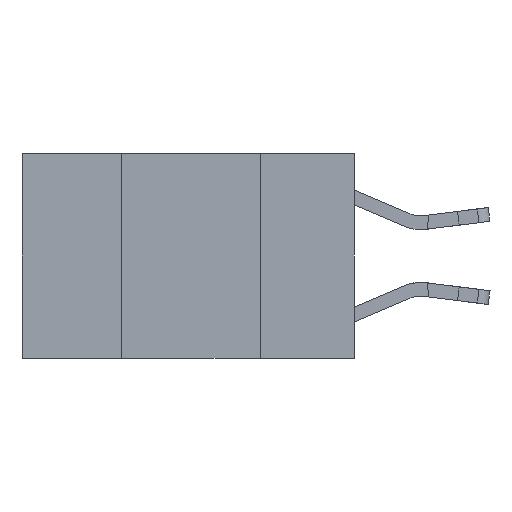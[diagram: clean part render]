
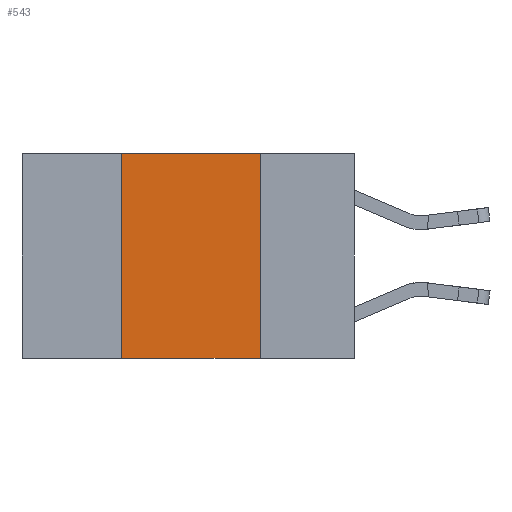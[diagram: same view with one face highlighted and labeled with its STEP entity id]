
A CAD part, left-side view. The second image highlights one B-rep face of the part: STEP entity #543.
In plain terms, the highlighted planar face has unit normal (-1, 0, 0).
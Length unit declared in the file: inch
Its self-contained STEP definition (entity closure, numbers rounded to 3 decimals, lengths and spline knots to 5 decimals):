
#543 = ADVANCED_FACE ( 'NONE', ( #21779 ), #15109, .F. ) ;
#1077 = CARTESIAN_POINT ( 'NONE',  ( 0., 0.42, -0.37 ) ) ;
#1255 = CARTESIAN_POINT ( 'NONE',  ( 0., 0.42, 0. ) ) ;
#1808 = LINE ( 'NONE', #9830, #12783 ) ;
#3515 = DIRECTION ( 'NONE',  ( 0., 0., -1. ) ) ;
#4391 = VECTOR ( 'NONE', #8949, 39.37008 ) ;
#5004 = VERTEX_POINT ( 'NONE', #21701 ) ;
#8763 = DIRECTION ( 'NONE',  ( 0., -1., 0. ) ) ;
#8823 = VERTEX_POINT ( 'NONE', #22672 ) ;
#8858 = CARTESIAN_POINT ( 'NONE',  ( 0., 0.42, 0. ) ) ;
#8949 = DIRECTION ( 'NONE',  ( 0., 0., 1. ) ) ;
#9587 = EDGE_CURVE ( 'NONE', #20659, #5004, #15775, .T. ) ;
#9830 = CARTESIAN_POINT ( 'NONE',  ( 0., 0.17, 0. ) ) ;
#10849 = CARTESIAN_POINT ( 'NONE',  ( 0., 0.6, -0.37 ) ) ;
#11234 = EDGE_LOOP ( 'NONE', ( #11750, #12379, #17799, #13031 ) ) ;
#11750 = ORIENTED_EDGE ( 'NONE', *, *, #12477, .F. ) ;
#12379 = ORIENTED_EDGE ( 'NONE', *, *, #22537, .F. ) ;
#12477 = EDGE_CURVE ( 'NONE', #8823, #5004, #1808, .T. ) ;
#12783 = VECTOR ( 'NONE', #3515, 39.37008 ) ;
#13031 = ORIENTED_EDGE ( 'NONE', *, *, #9587, .T. ) ;
#15109 = PLANE ( 'NONE',  #18834 ) ;
#15480 = CARTESIAN_POINT ( 'NONE',  ( 0., 0.6, 0. ) ) ;
#15775 = LINE ( 'NONE', #10849, #24631 ) ;
#15976 = LINE ( 'NONE', #8858, #4391 ) ;
#16313 = DIRECTION ( 'NONE',  ( 1., 0., 0. ) ) ;
#16536 = DIRECTION ( 'NONE',  ( 0., 0., -1. ) ) ;
#17236 = EDGE_CURVE ( 'NONE', #20659, #22680, #15976, .T. ) ;
#17799 = ORIENTED_EDGE ( 'NONE', *, *, #17236, .F. ) ;
#18834 = AXIS2_PLACEMENT_3D ( 'NONE', #15480, #16313, #16536 ) ;
#20659 = VERTEX_POINT ( 'NONE', #1077 ) ;
#21701 = CARTESIAN_POINT ( 'NONE',  ( 0., 0.17, -0.37 ) ) ;
#21779 = FACE_OUTER_BOUND ( 'NONE', #11234, .T. ) ;
#22537 = EDGE_CURVE ( 'NONE', #22680, #8823, #24919, .T. ) ;
#22672 = CARTESIAN_POINT ( 'NONE',  ( 0., 0.17, 0. ) ) ;
#22680 = VERTEX_POINT ( 'NONE', #1255 ) ;
#23354 = CARTESIAN_POINT ( 'NONE',  ( 0., 0.6, 0. ) ) ;
#24295 = VECTOR ( 'NONE', #25391, 39.37008 ) ;
#24631 = VECTOR ( 'NONE', #8763, 39.37008 ) ;
#24919 = LINE ( 'NONE', #23354, #24295 ) ;
#25391 = DIRECTION ( 'NONE',  ( 0., -1., 0. ) ) ;
